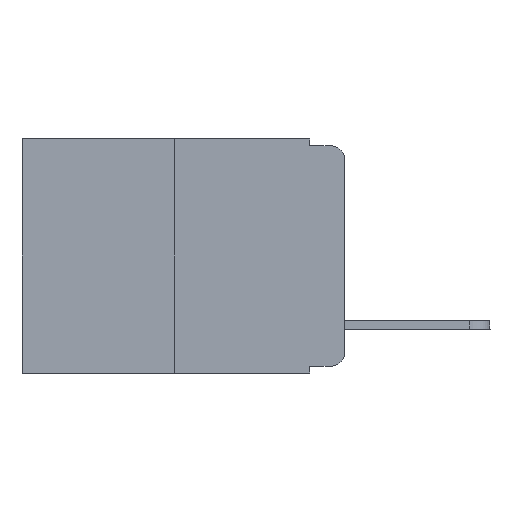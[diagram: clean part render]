
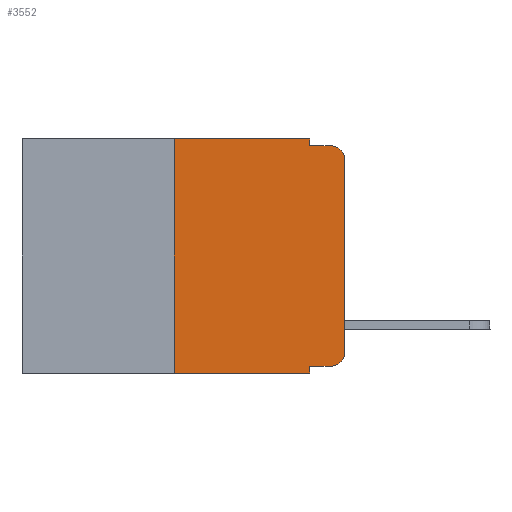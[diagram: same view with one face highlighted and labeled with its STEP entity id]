
A CAD part, left-side view. The second image highlights one B-rep face of the part: STEP entity #3552.
In plain terms, the highlighted planar face has unit normal (-1, 0, 0).
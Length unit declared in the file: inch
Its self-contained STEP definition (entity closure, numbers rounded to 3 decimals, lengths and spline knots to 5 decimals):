
#162 = DIRECTION ( 'NONE',  ( 0., 0., -1. ) ) ;
#516 = DIRECTION ( 'NONE',  ( 0., -1., 0. ) ) ;
#1474 = CARTESIAN_POINT ( 'NONE',  ( 0., 0.051, 0. ) ) ;
#1516 = EDGE_CURVE ( 'NONE', #2094, #5505, #10721, .T. ) ;
#1584 = VERTEX_POINT ( 'NONE', #13552 ) ;
#1768 = VERTEX_POINT ( 'NONE', #4409 ) ;
#1825 = VECTOR ( 'NONE', #8621, 39.37008 ) ;
#2051 = CARTESIAN_POINT ( 'NONE',  ( 0., 0.02, -0.03 ) ) ;
#2068 = CARTESIAN_POINT ( 'NONE',  ( 0., 0.051, -0.333 ) ) ;
#2094 = VERTEX_POINT ( 'NONE', #5061 ) ;
#2237 = ORIENTED_EDGE ( 'NONE', *, *, #2912, .T. ) ;
#2255 = LINE ( 'NONE', #2068, #14584 ) ;
#2550 = CARTESIAN_POINT ( 'NONE',  ( 0., 0.473, 0. ) ) ;
#2730 = LINE ( 'NONE', #17193, #13320 ) ;
#2912 = EDGE_CURVE ( 'NONE', #1584, #19144, #14414, .T. ) ;
#3070 = DIRECTION ( 'NONE',  ( 0., -1., 0. ) ) ;
#3195 = CARTESIAN_POINT ( 'NONE',  ( 0., 0.473, 0. ) ) ;
#3552 = ADVANCED_FACE ( 'NONE', ( #8228 ), #14206, .F. ) ;
#4098 = EDGE_CURVE ( 'NONE', #17734, #19144, #4332, .T. ) ;
#4167 = AXIS2_PLACEMENT_3D ( 'NONE', #11678, #7283, #162 ) ;
#4332 = LINE ( 'NONE', #16170, #18595 ) ;
#4409 = CARTESIAN_POINT ( 'NONE',  ( 0., 0.051, -0.343 ) ) ;
#4417 = VERTEX_POINT ( 'NONE', #7067 ) ;
#4952 = ORIENTED_EDGE ( 'NONE', *, *, #10814, .T. ) ;
#5061 = CARTESIAN_POINT ( 'NONE',  ( 0., 0.25, 0. ) ) ;
#5093 = CARTESIAN_POINT ( 'NONE',  ( 0., 0.25, -0.343 ) ) ;
#5109 = DIRECTION ( 'NONE',  ( -1., 0., 0. ) ) ;
#5290 = ORIENTED_EDGE ( 'NONE', *, *, #16661, .F. ) ;
#5505 = VERTEX_POINT ( 'NONE', #12110 ) ;
#5896 = CARTESIAN_POINT ( 'NONE',  ( 0., 0.02, -0.333 ) ) ;
#6241 = DIRECTION ( 'NONE',  ( 0., -1., 0. ) ) ;
#6716 = VECTOR ( 'NONE', #8898, 39.37008 ) ;
#7035 = DIRECTION ( 'NONE',  ( 0., 0., 1. ) ) ;
#7067 = CARTESIAN_POINT ( 'NONE',  ( 0., 0., -0.313 ) ) ;
#7176 = VECTOR ( 'NONE', #3070, 39.37008 ) ;
#7283 = DIRECTION ( 'NONE',  ( -1., 0., 0. ) ) ;
#7511 = VERTEX_POINT ( 'NONE', #5093 ) ;
#7610 = ORIENTED_EDGE ( 'NONE', *, *, #16160, .F. ) ;
#8228 = FACE_OUTER_BOUND ( 'NONE', #11566, .T. ) ;
#8557 = CARTESIAN_POINT ( 'NONE',  ( 0., 0.051, -0.333 ) ) ;
#8598 = CARTESIAN_POINT ( 'NONE',  ( 0., 0.051, -0.01 ) ) ;
#8621 = DIRECTION ( 'NONE',  ( 0., 0., -1. ) ) ;
#8898 = DIRECTION ( 'NONE',  ( 0., 0., -1. ) ) ;
#9423 = CIRCLE ( 'NONE', #4167, 0.02 ) ;
#10135 = EDGE_CURVE ( 'NONE', #11725, #13910, #2255, .T. ) ;
#10414 = LINE ( 'NONE', #16356, #7176 ) ;
#10721 = LINE ( 'NONE', #3195, #10922 ) ;
#10814 = EDGE_CURVE ( 'NONE', #7511, #1768, #10414, .T. ) ;
#10922 = VECTOR ( 'NONE', #6241, 39.37008 ) ;
#10964 = CARTESIAN_POINT ( 'NONE',  ( 0., 0.25, 0. ) ) ;
#11059 = DIRECTION ( 'NONE',  ( 0., 0., 1. ) ) ;
#11249 = CARTESIAN_POINT ( 'NONE',  ( 0., 0.02, -0.01 ) ) ;
#11566 = EDGE_LOOP ( 'NONE', ( #16912, #2237, #15044, #5290, #12784, #13102, #4952, #7610, #15070, #13689 ) ) ;
#11678 = CARTESIAN_POINT ( 'NONE',  ( 0., 0.02, -0.313 ) ) ;
#11725 = VERTEX_POINT ( 'NONE', #8557 ) ;
#11880 = EDGE_CURVE ( 'NONE', #13910, #4417, #9423, .T. ) ;
#12110 = CARTESIAN_POINT ( 'NONE',  ( 0., 0.051, 0. ) ) ;
#12578 = DIRECTION ( 'NONE',  ( 0., 0., -1. ) ) ;
#12614 = DIRECTION ( 'NONE',  ( 1., 0., 0. ) ) ;
#12784 = ORIENTED_EDGE ( 'NONE', *, *, #1516, .F. ) ;
#13078 = LINE ( 'NONE', #1474, #6716 ) ;
#13102 = ORIENTED_EDGE ( 'NONE', *, *, #17634, .F. ) ;
#13104 = CARTESIAN_POINT ( 'NONE',  ( 0., 0.051, 0. ) ) ;
#13320 = VECTOR ( 'NONE', #7035, 39.37008 ) ;
#13472 = AXIS2_PLACEMENT_3D ( 'NONE', #2051, #5109, #12578 ) ;
#13552 = CARTESIAN_POINT ( 'NONE',  ( 0., 0., -0.03 ) ) ;
#13609 = VECTOR ( 'NONE', #11059, 39.37008 ) ;
#13689 = ORIENTED_EDGE ( 'NONE', *, *, #11880, .T. ) ;
#13910 = VERTEX_POINT ( 'NONE', #5896 ) ;
#14206 = PLANE ( 'NONE',  #16949 ) ;
#14414 = CIRCLE ( 'NONE', #13472, 0.02 ) ;
#14584 = VECTOR ( 'NONE', #516, 39.37008 ) ;
#15044 = ORIENTED_EDGE ( 'NONE', *, *, #4098, .F. ) ;
#15070 = ORIENTED_EDGE ( 'NONE', *, *, #10135, .T. ) ;
#15850 = LINE ( 'NONE', #13104, #1825 ) ;
#16160 = EDGE_CURVE ( 'NONE', #11725, #1768, #15850, .T. ) ;
#16170 = CARTESIAN_POINT ( 'NONE',  ( 0., 0.051, -0.01 ) ) ;
#16356 = CARTESIAN_POINT ( 'NONE',  ( 0., 0.473, -0.343 ) ) ;
#16661 = EDGE_CURVE ( 'NONE', #5505, #17734, #13078, .T. ) ;
#16912 = ORIENTED_EDGE ( 'NONE', *, *, #19154, .T. ) ;
#16949 = AXIS2_PLACEMENT_3D ( 'NONE', #2550, #12614, #18476 ) ;
#17193 = CARTESIAN_POINT ( 'NONE',  ( 0., 0., 0. ) ) ;
#17634 = EDGE_CURVE ( 'NONE', #7511, #2094, #18365, .T. ) ;
#17734 = VERTEX_POINT ( 'NONE', #8598 ) ;
#18024 = DIRECTION ( 'NONE',  ( 0., -1., 0. ) ) ;
#18365 = LINE ( 'NONE', #10964, #13609 ) ;
#18476 = DIRECTION ( 'NONE',  ( 0., 0., -1. ) ) ;
#18595 = VECTOR ( 'NONE', #18024, 39.37008 ) ;
#19144 = VERTEX_POINT ( 'NONE', #11249 ) ;
#19154 = EDGE_CURVE ( 'NONE', #4417, #1584, #2730, .T. ) ;
